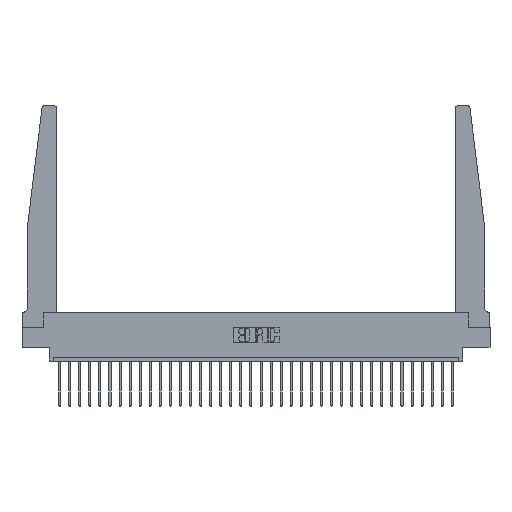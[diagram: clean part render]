
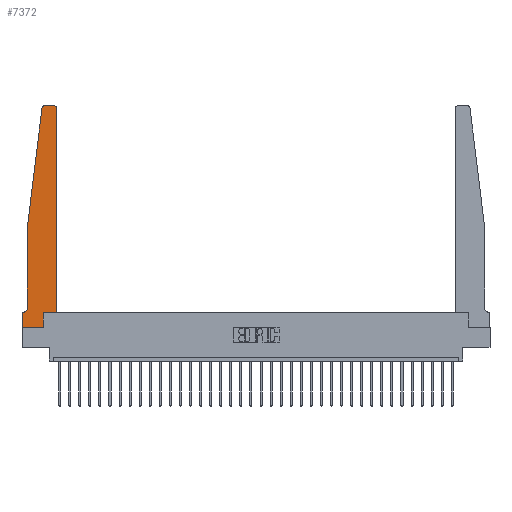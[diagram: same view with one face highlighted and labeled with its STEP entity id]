
A CAD part, top view. The second image highlights one B-rep face of the part: STEP entity #7372.
In plain terms, the highlighted planar face has unit normal (0, 0, 1).
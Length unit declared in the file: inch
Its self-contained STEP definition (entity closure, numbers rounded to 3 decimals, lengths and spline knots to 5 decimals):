
#484 = ORIENTED_EDGE ( 'NONE', *, *, #2826, .T. ) ;
#648 = CARTESIAN_POINT ( 'NONE',  ( 0.2605, 0., 0.37 ) ) ;
#1189 = EDGE_CURVE ( 'NONE', #24567, #9897, #17787, .T. ) ;
#1313 = ORIENTED_EDGE ( 'NONE', *, *, #22646, .T. ) ;
#1436 = CARTESIAN_POINT ( 'NONE',  ( 0., 0.1875, 0.37 ) ) ;
#1616 = VECTOR ( 'NONE', #18657, 39.37008 ) ;
#1858 = DIRECTION ( 'NONE',  ( 1., 0., 0. ) ) ;
#2207 = DIRECTION ( 'NONE',  ( -1., 0., 0. ) ) ;
#2282 = VERTEX_POINT ( 'NONE', #6344 ) ;
#2511 = CARTESIAN_POINT ( 'NONE',  ( 0.425, 2.72, 0.37 ) ) ;
#2826 = EDGE_CURVE ( 'NONE', #4110, #15959, #29464, .T. ) ;
#3596 = CARTESIAN_POINT ( 'NONE',  ( 0.425, 0.18, 0.37 ) ) ;
#3776 = EDGE_CURVE ( 'NONE', #15972, #19887, #20335, .T. ) ;
#4110 = VERTEX_POINT ( 'NONE', #7485 ) ;
#4221 = FACE_OUTER_BOUND ( 'NONE', #27323, .T. ) ;
#4605 = CARTESIAN_POINT ( 'NONE',  ( 0.425, 0.18, 0.37 ) ) ;
#4611 = CARTESIAN_POINT ( 'NONE',  ( 0.065, 1.25, 0.37 ) ) ;
#4616 = DIRECTION ( 'NONE',  ( 0., 0., 1. ) ) ;
#4944 = EDGE_CURVE ( 'NONE', #10570, #22477, #14131, .T. ) ;
#5547 = CARTESIAN_POINT ( 'NONE',  ( 0.27653, 2.72, 0.37 ) ) ;
#5635 = CARTESIAN_POINT ( 'NONE',  ( 0.015, 0.2375, 0.37 ) ) ;
#5657 = ORIENTED_EDGE ( 'NONE', *, *, #25511, .T. ) ;
#6238 = DIRECTION ( 'NONE',  ( -1., 0., 0. ) ) ;
#6344 = CARTESIAN_POINT ( 'NONE',  ( 0.015, 0.1875, 0.37 ) ) ;
#6533 = EDGE_CURVE ( 'NONE', #22477, #22257, #19137, .T. ) ;
#6749 = AXIS2_PLACEMENT_3D ( 'NONE', #5635, #7992, #10914 ) ;
#7095 = VERTEX_POINT ( 'NONE', #28059 ) ;
#7372 = ADVANCED_FACE ( 'NONE', ( #4221 ), #27332, .T. ) ;
#7485 = CARTESIAN_POINT ( 'NONE',  ( 0.065, 1.25, 0.37 ) ) ;
#7524 = LINE ( 'NONE', #12967, #18375 ) ;
#7802 = LINE ( 'NONE', #29054, #16448 ) ;
#7842 = VECTOR ( 'NONE', #15858, 39.37008 ) ;
#7881 = DIRECTION ( 'NONE',  ( 0., 1., 0. ) ) ;
#7992 = DIRECTION ( 'NONE',  ( 0., 0., -1. ) ) ;
#8045 = VECTOR ( 'NONE', #23475, 39.37008 ) ;
#8382 = CARTESIAN_POINT ( 'NONE',  ( 0.2605, 0.18, 0.37 ) ) ;
#8662 = CIRCLE ( 'NONE', #20320, 0.03 ) ;
#8842 = DIRECTION ( 'NONE',  ( 1., 0., 0. ) ) ;
#9139 = CARTESIAN_POINT ( 'NONE',  ( 0.065, 0.2375, 0.37 ) ) ;
#9897 = VERTEX_POINT ( 'NONE', #4605 ) ;
#10028 = DIRECTION ( 'NONE',  ( 1., 0., 0. ) ) ;
#10570 = VERTEX_POINT ( 'NONE', #2511 ) ;
#10914 = DIRECTION ( 'NONE',  ( -1., 0., 0. ) ) ;
#11477 = DIRECTION ( 'NONE',  ( 1., 0., 0. ) ) ;
#11646 = CARTESIAN_POINT ( 'NONE',  ( 0.2605, 0.18, 0.37 ) ) ;
#12030 = EDGE_CURVE ( 'NONE', #25153, #15972, #28562, .T. ) ;
#12052 = VECTOR ( 'NONE', #8842, 39.37008 ) ;
#12266 = DIRECTION ( 'NONE',  ( 0., 0., 1. ) ) ;
#12331 = EDGE_CURVE ( 'NONE', #22257, #7095, #8662, .T. ) ;
#12967 = CARTESIAN_POINT ( 'NONE',  ( 0.065, 0.1875, 0.37 ) ) ;
#13515 = CARTESIAN_POINT ( 'NONE',  ( 0.395, 2.75, 0.37 ) ) ;
#13585 = ORIENTED_EDGE ( 'NONE', *, *, #12030, .T. ) ;
#13714 = ORIENTED_EDGE ( 'NONE', *, *, #1189, .T. ) ;
#14032 = ORIENTED_EDGE ( 'NONE', *, *, #18786, .T. ) ;
#14131 = CIRCLE ( 'NONE', #29814, 0.03 ) ;
#14239 = CARTESIAN_POINT ( 'NONE',  ( 0.27653, 2.75, 0.37 ) ) ;
#14543 = EDGE_CURVE ( 'NONE', #9897, #10570, #7802, .T. ) ;
#15435 = CARTESIAN_POINT ( 'NONE',  ( 0.065, 1.25, 0.37 ) ) ;
#15707 = CARTESIAN_POINT ( 'NONE',  ( 0.395, 2.72, 0.37 ) ) ;
#15858 = DIRECTION ( 'NONE',  ( -0.122, -0.992, 0. ) ) ;
#15954 = CARTESIAN_POINT ( 'NONE',  ( 0.25, 2.75, 0.37 ) ) ;
#15959 = VERTEX_POINT ( 'NONE', #9139 ) ;
#15972 = VERTEX_POINT ( 'NONE', #20946 ) ;
#16448 = VECTOR ( 'NONE', #7881, 39.37008 ) ;
#16891 = ORIENTED_EDGE ( 'NONE', *, *, #14543, .T. ) ;
#17064 = DIRECTION ( 'NONE',  ( 0., -1., 0. ) ) ;
#17787 = LINE ( 'NONE', #3596, #12052 ) ;
#18249 = AXIS2_PLACEMENT_3D ( 'NONE', #1436, #4616, #11477 ) ;
#18375 = VECTOR ( 'NONE', #6238, 39.37008 ) ;
#18657 = DIRECTION ( 'NONE',  ( 0., -1., 0. ) ) ;
#18786 = EDGE_CURVE ( 'NONE', #2282, #25153, #7524, .T. ) ;
#19137 = LINE ( 'NONE', #15954, #20914 ) ;
#19498 = ORIENTED_EDGE ( 'NONE', *, *, #25346, .T. ) ;
#19595 = VECTOR ( 'NONE', #23062, 39.37008 ) ;
#19887 = VERTEX_POINT ( 'NONE', #648 ) ;
#20320 = AXIS2_PLACEMENT_3D ( 'NONE', #5547, #12266, #10028 ) ;
#20335 = LINE ( 'NONE', #23267, #8045 ) ;
#20349 = ORIENTED_EDGE ( 'NONE', *, *, #6533, .T. ) ;
#20464 = CIRCLE ( 'NONE', #6749, 0.05 ) ;
#20914 = VECTOR ( 'NONE', #2207, 39.37008 ) ;
#20946 = CARTESIAN_POINT ( 'NONE',  ( 0., 0., 0.37 ) ) ;
#21036 = CARTESIAN_POINT ( 'NONE',  ( 0., 0.1875, 0.37 ) ) ;
#22257 = VERTEX_POINT ( 'NONE', #14239 ) ;
#22477 = VERTEX_POINT ( 'NONE', #13515 ) ;
#22620 = ORIENTED_EDGE ( 'NONE', *, *, #4944, .T. ) ;
#22646 = EDGE_CURVE ( 'NONE', #19887, #24567, #24997, .T. ) ;
#23062 = DIRECTION ( 'NONE',  ( 0., 1., 0. ) ) ;
#23267 = CARTESIAN_POINT ( 'NONE',  ( 0., 0., 0.37 ) ) ;
#23475 = DIRECTION ( 'NONE',  ( 1., 0., 0. ) ) ;
#24567 = VERTEX_POINT ( 'NONE', #8382 ) ;
#24790 = ORIENTED_EDGE ( 'NONE', *, *, #3776, .T. ) ;
#24997 = LINE ( 'NONE', #11646, #19595 ) ;
#25094 = DIRECTION ( 'NONE',  ( 0., 0., 1. ) ) ;
#25153 = VERTEX_POINT ( 'NONE', #21036 ) ;
#25346 = EDGE_CURVE ( 'NONE', #15959, #2282, #20464, .T. ) ;
#25511 = EDGE_CURVE ( 'NONE', #7095, #4110, #26293, .T. ) ;
#26293 = LINE ( 'NONE', #4611, #7842 ) ;
#26307 = CARTESIAN_POINT ( 'NONE',  ( 0., 0., 0.37 ) ) ;
#27323 = EDGE_LOOP ( 'NONE', ( #20349, #29195, #5657, #484, #19498, #14032, #13585, #24790, #1313, #13714, #16891, #22620 ) ) ;
#27332 = PLANE ( 'NONE',  #18249 ) ;
#27848 = VECTOR ( 'NONE', #17064, 39.37008 ) ;
#28059 = CARTESIAN_POINT ( 'NONE',  ( 0.24675, 2.72367, 0.37 ) ) ;
#28562 = LINE ( 'NONE', #26307, #27848 ) ;
#29054 = CARTESIAN_POINT ( 'NONE',  ( 0.425, 0.18, 0.37 ) ) ;
#29195 = ORIENTED_EDGE ( 'NONE', *, *, #12331, .T. ) ;
#29464 = LINE ( 'NONE', #15435, #1616 ) ;
#29814 = AXIS2_PLACEMENT_3D ( 'NONE', #15707, #25094, #1858 ) ;
